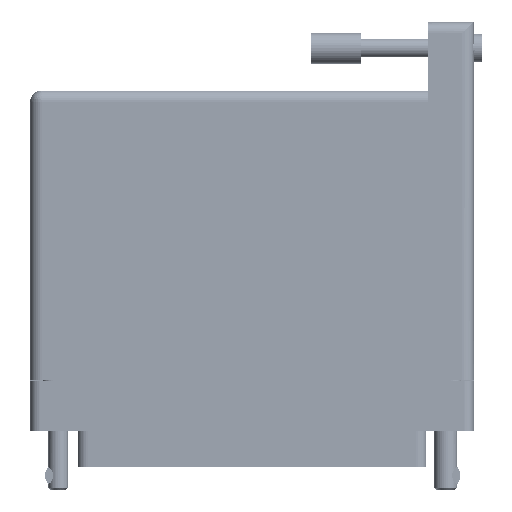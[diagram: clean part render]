
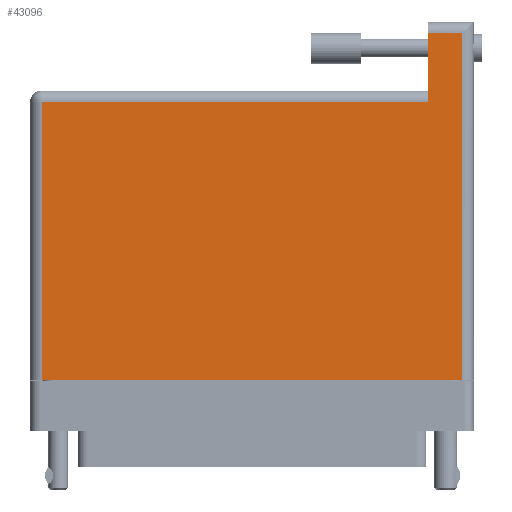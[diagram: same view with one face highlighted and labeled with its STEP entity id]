
A CAD part, front view. The second image highlights one B-rep face of the part: STEP entity #43096.
In plain terms, the highlighted face is planar.
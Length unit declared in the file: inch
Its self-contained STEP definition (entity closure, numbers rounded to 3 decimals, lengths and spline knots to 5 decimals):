
#146 = DIRECTION ( 'NONE',  ( 0., -1., 0. ) ) ;
#641 = FACE_OUTER_BOUND ( 'NONE', #42687, .T. ) ;
#1796 = DIRECTION ( 'NONE',  ( 0., 0., -1. ) ) ;
#1848 = VERTEX_POINT ( 'NONE', #78131 ) ;
#2339 = ORIENTED_EDGE ( 'NONE', *, *, #54934, .T. ) ;
#2593 = EDGE_CURVE ( 'NONE', #82384, #67921, #30906, .T. ) ;
#3501 = LINE ( 'NONE', #59768, #4416 ) ;
#4416 = VECTOR ( 'NONE', #21012, 39.37008 ) ;
#4490 = DIRECTION ( 'NONE',  ( -1., 0., 0. ) ) ;
#5958 = VECTOR ( 'NONE', #18563, 39.37008 ) ;
#6732 = VERTEX_POINT ( 'NONE', #44755 ) ;
#7009 = VECTOR ( 'NONE', #4490, 39.37008 ) ;
#8016 = PLANE ( 'NONE',  #68851 ) ;
#8305 = DIRECTION ( 'NONE',  ( -1., 0., 0. ) ) ;
#9503 = LINE ( 'NONE', #25313, #40778 ) ;
#11739 = VECTOR ( 'NONE', #47207, 39.37008 ) ;
#12035 = EDGE_CURVE ( 'NONE', #37886, #74765, #24212, .T. ) ;
#14460 = CARTESIAN_POINT ( 'NONE',  ( 1.289, -0.1, 0.617 ) ) ;
#17216 = CARTESIAN_POINT ( 'NONE',  ( -1.289, 1.605, 0.617 ) ) ;
#17580 = ORIENTED_EDGE ( 'NONE', *, *, #12035, .T. ) ;
#18563 = DIRECTION ( 'NONE',  ( 0., -1., 0. ) ) ;
#19262 = CARTESIAN_POINT ( 'NONE',  ( 1.079, 1.605, 0.617 ) ) ;
#21012 = DIRECTION ( 'NONE',  ( 0., 1., 0. ) ) ;
#22652 = ORIENTED_EDGE ( 'NONE', *, *, #2593, .T. ) ;
#24212 = LINE ( 'NONE', #55088, #7009 ) ;
#25313 = CARTESIAN_POINT ( 'NONE',  ( -1.289, -0.1, 0.617 ) ) ;
#30361 = CARTESIAN_POINT ( 'NONE',  ( 1.079, 2.095, 0.617 ) ) ;
#30906 = LINE ( 'NONE', #60509, #11739 ) ;
#32641 = VECTOR ( 'NONE', #63832, 39.37008 ) ;
#37886 = VERTEX_POINT ( 'NONE', #19262 ) ;
#38405 = ORIENTED_EDGE ( 'NONE', *, *, #60019, .T. ) ;
#40386 = LINE ( 'NONE', #30361, #5958 ) ;
#40778 = VECTOR ( 'NONE', #146, 39.37008 ) ;
#42687 = EDGE_LOOP ( 'NONE', ( #17580, #73276, #22652, #45564, #38405, #2339 ) ) ;
#43096 = ADVANCED_FACE ( 'NONE', ( #641 ), #8016, .F. ) ;
#44755 = CARTESIAN_POINT ( 'NONE',  ( 1.289, 2.025, 0.617 ) ) ;
#45564 = ORIENTED_EDGE ( 'NONE', *, *, #48389, .T. ) ;
#47207 = DIRECTION ( 'NONE',  ( 1., 0., 0. ) ) ;
#48389 = EDGE_CURVE ( 'NONE', #67921, #6732, #3501, .T. ) ;
#54934 = EDGE_CURVE ( 'NONE', #1848, #37886, #40386, .T. ) ;
#55088 = CARTESIAN_POINT ( 'NONE',  ( -1.359, 1.605, 0.617 ) ) ;
#55452 = CARTESIAN_POINT ( 'NONE',  ( -1.289, -0.1, 0.617 ) ) ;
#59768 = CARTESIAN_POINT ( 'NONE',  ( 1.289, 2.095, 0.617 ) ) ;
#60019 = EDGE_CURVE ( 'NONE', #6732, #1848, #63051, .T. ) ;
#60509 = CARTESIAN_POINT ( 'NONE',  ( -1.359, -0.1, 0.617 ) ) ;
#63051 = LINE ( 'NONE', #71387, #32641 ) ;
#63832 = DIRECTION ( 'NONE',  ( -1., 0., 0. ) ) ;
#67921 = VERTEX_POINT ( 'NONE', #14460 ) ;
#68851 = AXIS2_PLACEMENT_3D ( 'NONE', #79518, #1796, #8305 ) ;
#71387 = CARTESIAN_POINT ( 'NONE',  ( -1.359, 2.025, 0.617 ) ) ;
#73276 = ORIENTED_EDGE ( 'NONE', *, *, #77783, .T. ) ;
#74765 = VERTEX_POINT ( 'NONE', #17216 ) ;
#77783 = EDGE_CURVE ( 'NONE', #74765, #82384, #9503, .T. ) ;
#78131 = CARTESIAN_POINT ( 'NONE',  ( 1.079, 2.025, 0.617 ) ) ;
#79518 = CARTESIAN_POINT ( 'NONE',  ( -1.359, 1.675, 0.617 ) ) ;
#82384 = VERTEX_POINT ( 'NONE', #55452 ) ;
